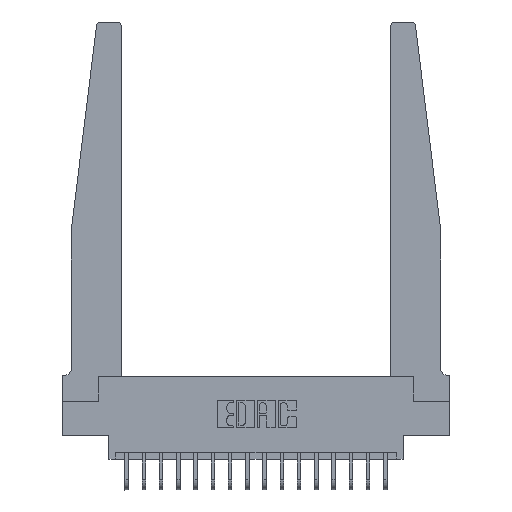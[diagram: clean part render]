
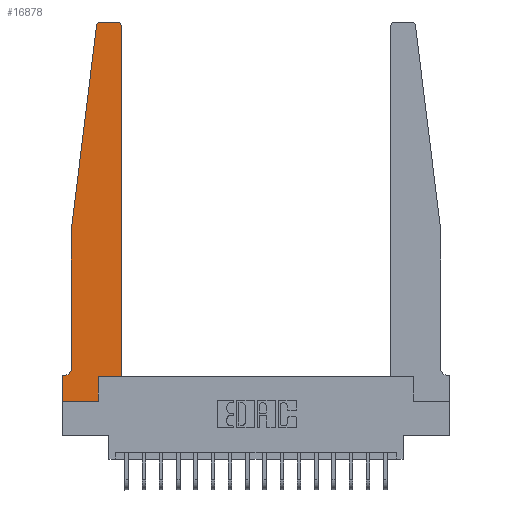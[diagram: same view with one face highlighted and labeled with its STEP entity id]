
A CAD part, top view. The second image highlights one B-rep face of the part: STEP entity #16878.
In plain terms, the highlighted planar face has unit normal (0, 0, 1).
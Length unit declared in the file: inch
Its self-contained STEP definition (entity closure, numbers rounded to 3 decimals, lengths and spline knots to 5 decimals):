
#370 = CARTESIAN_POINT ( 'NONE',  ( 0.015, 0.1875, 0.37 ) ) ;
#616 = LINE ( 'NONE', #4902, #1363 ) ;
#621 = ORIENTED_EDGE ( 'NONE', *, *, #9776, .T. ) ;
#1020 = CARTESIAN_POINT ( 'NONE',  ( 0.425, 0.18, 0.37 ) ) ;
#1043 = CARTESIAN_POINT ( 'NONE',  ( 0.425, 0.18, 0.37 ) ) ;
#1269 = EDGE_CURVE ( 'NONE', #2831, #18329, #19747, .T. ) ;
#1363 = VECTOR ( 'NONE', #19258, 39.37008 ) ;
#1636 = DIRECTION ( 'NONE',  ( -1., 0., 0. ) ) ;
#2330 = EDGE_CURVE ( 'NONE', #16164, #17940, #13205, .T. ) ;
#2530 = CARTESIAN_POINT ( 'NONE',  ( 0.065, 0.2375, 0.37 ) ) ;
#2618 = CARTESIAN_POINT ( 'NONE',  ( 0.015, 0.2375, 0.37 ) ) ;
#2748 = EDGE_CURVE ( 'NONE', #8474, #19734, #5699, .T. ) ;
#2831 = VERTEX_POINT ( 'NONE', #4056 ) ;
#2866 = DIRECTION ( 'NONE',  ( 0., -1., 0. ) ) ;
#3161 = LINE ( 'NONE', #15770, #19405 ) ;
#3219 = CARTESIAN_POINT ( 'NONE',  ( 0.27653, 2.72, 0.37 ) ) ;
#3495 = EDGE_CURVE ( 'NONE', #11314, #16164, #3913, .T. ) ;
#3913 = LINE ( 'NONE', #15287, #17407 ) ;
#4056 = CARTESIAN_POINT ( 'NONE',  ( 0.425, 2.72, 0.37 ) ) ;
#4081 = ORIENTED_EDGE ( 'NONE', *, *, #16206, .T. ) ;
#4309 = DIRECTION ( 'NONE',  ( 1., 0., 0. ) ) ;
#4421 = ORIENTED_EDGE ( 'NONE', *, *, #19321, .T. ) ;
#4444 = CARTESIAN_POINT ( 'NONE',  ( 0.2605, 0., 0.37 ) ) ;
#4585 = DIRECTION ( 'NONE',  ( 0., 0., 1. ) ) ;
#4680 = EDGE_LOOP ( 'NONE', ( #621, #11849, #7884, #15138, #4081, #5010, #13303, #16593, #4421, #19456, #10131, #5145 ) ) ;
#4691 = VERTEX_POINT ( 'NONE', #4444 ) ;
#4777 = VECTOR ( 'NONE', #12359, 39.37008 ) ;
#4902 = CARTESIAN_POINT ( 'NONE',  ( 0.065, 1.25, 0.37 ) ) ;
#5010 = ORIENTED_EDGE ( 'NONE', *, *, #3495, .T. ) ;
#5145 = ORIENTED_EDGE ( 'NONE', *, *, #1269, .T. ) ;
#5202 = VERTEX_POINT ( 'NONE', #16134 ) ;
#5312 = CARTESIAN_POINT ( 'NONE',  ( 0.425, 0.18, 0.37 ) ) ;
#5699 = LINE ( 'NONE', #5312, #12433 ) ;
#6134 = CARTESIAN_POINT ( 'NONE',  ( 0., 0., 0.37 ) ) ;
#6457 = DIRECTION ( 'NONE',  ( 0., 1., 0. ) ) ;
#6524 = LINE ( 'NONE', #1043, #11279 ) ;
#6539 = VECTOR ( 'NONE', #6457, 39.37008 ) ;
#6746 = EDGE_CURVE ( 'NONE', #19734, #2831, #6524, .T. ) ;
#6748 = CARTESIAN_POINT ( 'NONE',  ( 0.395, 2.75, 0.37 ) ) ;
#7092 = VERTEX_POINT ( 'NONE', #8617 ) ;
#7325 = DIRECTION ( 'NONE',  ( -1., 0., 0. ) ) ;
#7751 = DIRECTION ( 'NONE',  ( 1., 0., 0. ) ) ;
#7884 = ORIENTED_EDGE ( 'NONE', *, *, #13468, .T. ) ;
#8146 = VECTOR ( 'NONE', #14324, 39.37008 ) ;
#8474 = VERTEX_POINT ( 'NONE', #15817 ) ;
#8617 = CARTESIAN_POINT ( 'NONE',  ( 0.24675, 2.72367, 0.37 ) ) ;
#8884 = CIRCLE ( 'NONE', #12556, 0.03 ) ;
#8988 = LINE ( 'NONE', #13917, #4777 ) ;
#9776 = EDGE_CURVE ( 'NONE', #18329, #5202, #3161, .T. ) ;
#10131 = ORIENTED_EDGE ( 'NONE', *, *, #6746, .T. ) ;
#10344 = DIRECTION ( 'NONE',  ( -1., 0., 0. ) ) ;
#10739 = VERTEX_POINT ( 'NONE', #16484 ) ;
#10872 = PLANE ( 'NONE',  #12838 ) ;
#10937 = CARTESIAN_POINT ( 'NONE',  ( 0., 0.1875, 0.37 ) ) ;
#11279 = VECTOR ( 'NONE', #15247, 39.37008 ) ;
#11314 = VERTEX_POINT ( 'NONE', #370 ) ;
#11411 = CARTESIAN_POINT ( 'NONE',  ( 0.2605, 0.18, 0.37 ) ) ;
#11849 = ORIENTED_EDGE ( 'NONE', *, *, #16035, .T. ) ;
#12359 = DIRECTION ( 'NONE',  ( -0.122, -0.992, 0. ) ) ;
#12433 = VECTOR ( 'NONE', #18076, 39.37008 ) ;
#12556 = AXIS2_PLACEMENT_3D ( 'NONE', #3219, #14418, #7751 ) ;
#12838 = AXIS2_PLACEMENT_3D ( 'NONE', #10937, #18889, #18760 ) ;
#13205 = LINE ( 'NONE', #6134, #18446 ) ;
#13303 = ORIENTED_EDGE ( 'NONE', *, *, #2330, .T. ) ;
#13468 = EDGE_CURVE ( 'NONE', #7092, #10739, #8988, .T. ) ;
#13507 = DIRECTION ( 'NONE',  ( 0., 0., -1. ) ) ;
#13656 = AXIS2_PLACEMENT_3D ( 'NONE', #2618, #13507, #10344 ) ;
#13917 = CARTESIAN_POINT ( 'NONE',  ( 0.065, 1.25, 0.37 ) ) ;
#14182 = CIRCLE ( 'NONE', #13656, 0.05 ) ;
#14324 = DIRECTION ( 'NONE',  ( 1., 0., 0. ) ) ;
#14418 = DIRECTION ( 'NONE',  ( 0., 0., 1. ) ) ;
#14548 = LINE ( 'NONE', #11411, #6539 ) ;
#15138 = ORIENTED_EDGE ( 'NONE', *, *, #18289, .T. ) ;
#15247 = DIRECTION ( 'NONE',  ( 0., 1., 0. ) ) ;
#15287 = CARTESIAN_POINT ( 'NONE',  ( 0.065, 0.1875, 0.37 ) ) ;
#15770 = CARTESIAN_POINT ( 'NONE',  ( 0.25, 2.75, 0.37 ) ) ;
#15817 = CARTESIAN_POINT ( 'NONE',  ( 0.2605, 0.18, 0.37 ) ) ;
#16035 = EDGE_CURVE ( 'NONE', #5202, #7092, #8884, .T. ) ;
#16134 = CARTESIAN_POINT ( 'NONE',  ( 0.27653, 2.75, 0.37 ) ) ;
#16164 = VERTEX_POINT ( 'NONE', #16628 ) ;
#16206 = EDGE_CURVE ( 'NONE', #20295, #11314, #14182, .T. ) ;
#16418 = EDGE_CURVE ( 'NONE', #17940, #4691, #18663, .T. ) ;
#16484 = CARTESIAN_POINT ( 'NONE',  ( 0.065, 1.25, 0.37 ) ) ;
#16593 = ORIENTED_EDGE ( 'NONE', *, *, #16418, .T. ) ;
#16628 = CARTESIAN_POINT ( 'NONE',  ( 0., 0.1875, 0.37 ) ) ;
#16836 = CARTESIAN_POINT ( 'NONE',  ( 0., 0., 0.37 ) ) ;
#16878 = ADVANCED_FACE ( 'NONE', ( #20627 ), #10872, .T. ) ;
#17274 = CARTESIAN_POINT ( 'NONE',  ( 0.395, 2.72, 0.37 ) ) ;
#17381 = CARTESIAN_POINT ( 'NONE',  ( 0., 0., 0.37 ) ) ;
#17407 = VECTOR ( 'NONE', #7325, 39.37008 ) ;
#17940 = VERTEX_POINT ( 'NONE', #16836 ) ;
#18076 = DIRECTION ( 'NONE',  ( 1., 0., 0. ) ) ;
#18289 = EDGE_CURVE ( 'NONE', #10739, #20295, #616, .T. ) ;
#18329 = VERTEX_POINT ( 'NONE', #6748 ) ;
#18446 = VECTOR ( 'NONE', #2866, 39.37008 ) ;
#18663 = LINE ( 'NONE', #17381, #8146 ) ;
#18760 = DIRECTION ( 'NONE',  ( 1., 0., 0. ) ) ;
#18889 = DIRECTION ( 'NONE',  ( 0., 0., 1. ) ) ;
#19258 = DIRECTION ( 'NONE',  ( 0., -1., 0. ) ) ;
#19321 = EDGE_CURVE ( 'NONE', #4691, #8474, #14548, .T. ) ;
#19405 = VECTOR ( 'NONE', #1636, 39.37008 ) ;
#19456 = ORIENTED_EDGE ( 'NONE', *, *, #2748, .T. ) ;
#19734 = VERTEX_POINT ( 'NONE', #1020 ) ;
#19747 = CIRCLE ( 'NONE', #20018, 0.03 ) ;
#20018 = AXIS2_PLACEMENT_3D ( 'NONE', #17274, #4585, #4309 ) ;
#20295 = VERTEX_POINT ( 'NONE', #2530 ) ;
#20627 = FACE_OUTER_BOUND ( 'NONE', #4680, .T. ) ;
